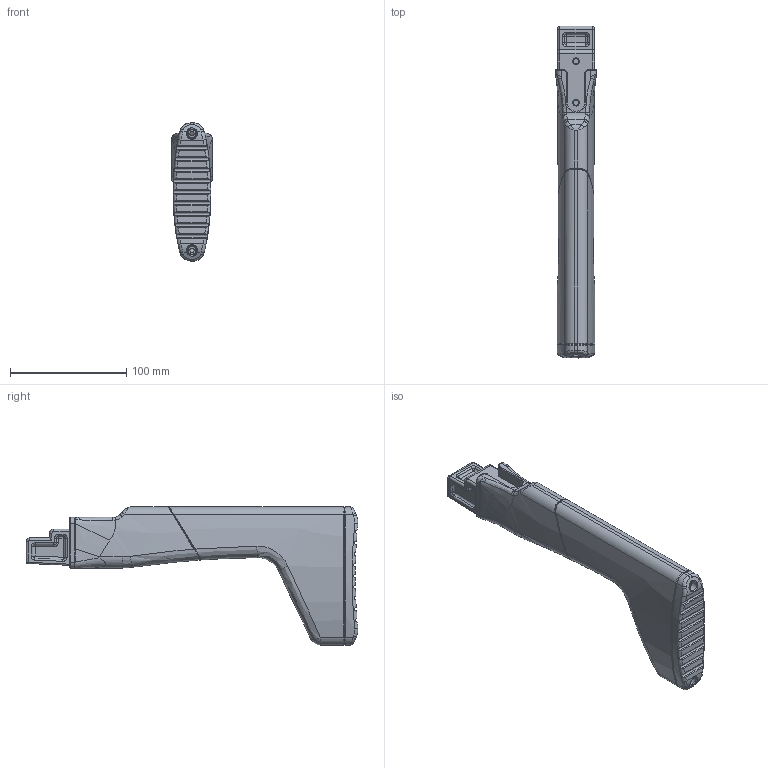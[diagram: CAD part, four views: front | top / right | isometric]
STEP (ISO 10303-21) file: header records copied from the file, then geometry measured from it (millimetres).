
FILE_DESCRIPTION(/* description */ (''),/* implementation_level */ '2;1');
FILE_NAME(/* name */ 'Spilt Stock.step',/* time_stamp */ '2021-10-03T07:00:48-04:00',/* author */ (''),/* organization */ (''),/* preprocessor_version */ 'ST-DEVELOPER v18.1',/* originating_system */ 'Autodesk Translation Framework v10.10.0.1391',/* authorisation */ '');
FILE_SCHEMA (('AUTOMOTIVE_DESIGN { 1 0 10303 214 3 1 1 }'));
Length unit declared in the file: millimetre
Products named in the file (1): 2 Part Stock
Bounding box: 35 x 285.01 x 118.61 mm (x, y, z)
Volume: 278590.5 mm3; surface area: 84835.4 mm2
Topology: 3 solids, 3 shells, 576 faces, 1325 edges, 774 vertices
Faces by surface type: bspline 237, cylinder 185, plane 69, torus 43, sphere 32, cone 10
Full cylindrical faces by diameter (mm): 1.952 x1, 2 x2, 3.8 x4, 4.6 x2, 6.7 x8, 8 x2
Entity records: 24422 total; most frequent: CARTESIAN_POINT 12704, ORIENTED_EDGE 2638, DIRECTION 2043, EDGE_CURVE 1319, AXIS2_PLACEMENT_3D 837, VERTEX_POINT 774, EDGE_LOOP 611, FACE_OUTER_BOUND 576
